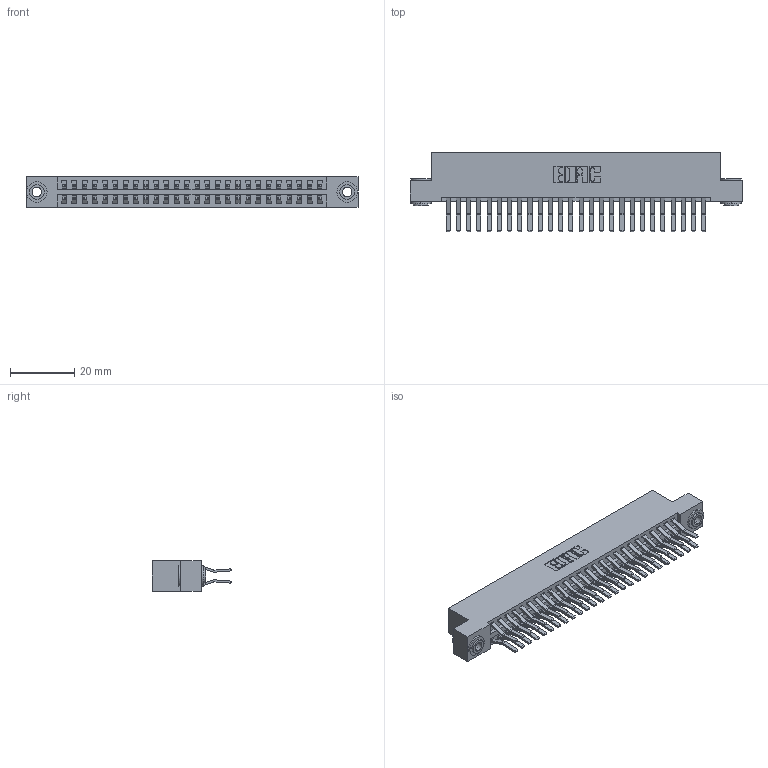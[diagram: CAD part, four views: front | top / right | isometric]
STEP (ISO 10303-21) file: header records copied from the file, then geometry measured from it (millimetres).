
FILE_DESCRIPTION (( 'STEP AP203' ), '1' );
FILE_NAME ('346-052-560-203.STEP', '2018-08-28T00:35:16', ( '' ), ( '' ), 'SwSTEP 2.0', 'SolidWorks 2016', '' );
FILE_SCHEMA (( 'CONFIG_CONTROL_DESIGN' ));
Length unit declared in the file: inch
Products named in the file (4): 345-250-002_345-250-002-102; 346-052-560-203; 346 Part_Flush Mounting Lugs - 0.156 Dia-TH; 345-292-001_560 Tail
Assembly tree (55 placements, depth 2):
  346-052-560-203
    346 Part_Flush Mounting Lugs - 0.156 Dia-TH
    345-292-001_560 Tail  x52
    345-250-002_345-250-002-102  x2
Bounding box: 103.12 x 24.78 x 9.4 mm (x, y, z)
Volume: 10291.8 mm3; surface area: 15018.9 mm2
Topology: 55 solids, 55 shells, 2968 faces, 8777 edges, 5778 vertices
Faces by surface type: plane 1906, cylinder 1054, cone 8
Entity records: 19860 total; most frequent: CARTESIAN_POINT 3271, ORIENTED_EDGE 3198, DIRECTION 2969, EDGE_CURVE 1599, LINE 1335, VECTOR 1335, VERTEX_POINT 1062, AXIS2_PLACEMENT_3D 817
